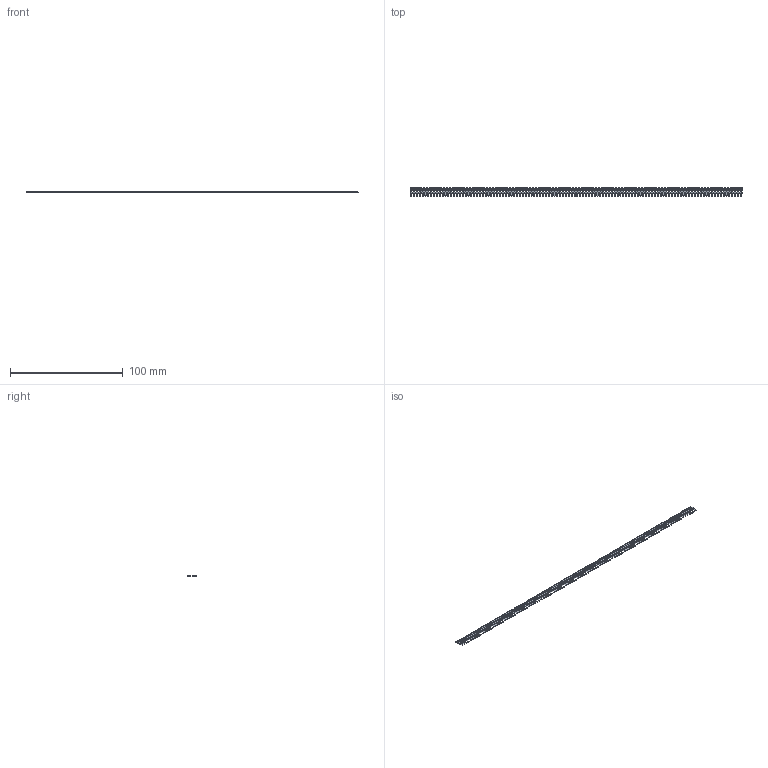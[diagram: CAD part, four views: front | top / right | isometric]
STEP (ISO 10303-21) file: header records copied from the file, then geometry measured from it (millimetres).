
FILE_DESCRIPTION (( 'STEP AP203' ), '1' );
FILE_NAME ('103-116-253-100.STEP', '2020-04-16T17:34:24', ( '' ), ( '' ), 'SwSTEP 2.0', 'SolidWorks 2016', '' );
FILE_SCHEMA (( 'CONFIG_CONTROL_DESIGN' ));
Length unit declared in the file: inch
Products named in the file (2): 103-116-253-100; 100-290-001_100-290-253
Assembly tree (116 placements, depth 2):
  103-116-253-100
    100-290-001_100-290-253  x116
Bounding box: 294.13 x 7.62 x 0.51 mm (x, y, z)
Volume: 640 mm3; surface area: 3991.2 mm2
Topology: 116 solids, 116 shells, 2320 faces, 6264 edges, 4176 vertices
Faces by surface type: plane 2204, cylinder 116
Entity records: 4500 total; most frequent: DIRECTION 334, COORDINATED_UNIVERSAL_TIME_OFFSET 242, LOCAL_TIME 242, DATE_AND_TIME 242, CALENDAR_DATE 242, CARTESIAN_POINT 229, AXIS2_PLACEMENT_3D 141, PERSON_AND_ORGANIZATION 132
